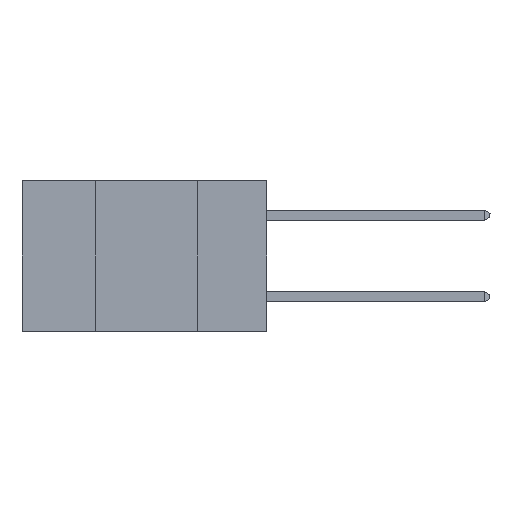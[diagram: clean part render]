
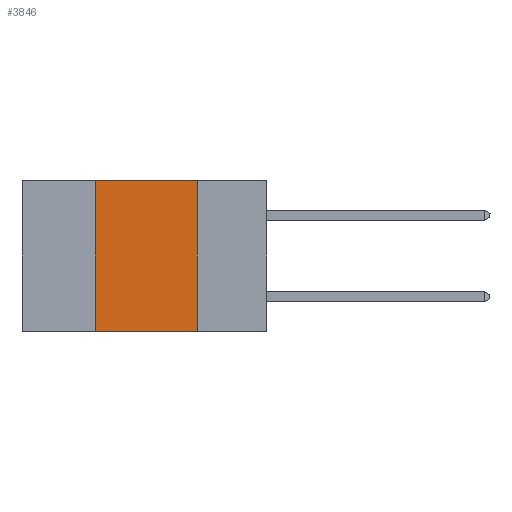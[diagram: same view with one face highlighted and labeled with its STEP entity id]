
A CAD part, left-side view. The second image highlights one B-rep face of the part: STEP entity #3846.
In plain terms, the highlighted planar face has unit normal (-1, 0, 0).
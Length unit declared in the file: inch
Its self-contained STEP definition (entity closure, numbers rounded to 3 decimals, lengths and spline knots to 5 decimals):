
#705 = VECTOR ( 'NONE', #15001, 39.37008 ) ;
#826 = PLANE ( 'NONE',  #18335 ) ;
#1712 = VECTOR ( 'NONE', #2984, 39.37008 ) ;
#1900 = DIRECTION ( 'NONE',  ( 0., -1., 0. ) ) ;
#2790 = VERTEX_POINT ( 'NONE', #8900 ) ;
#2984 = DIRECTION ( 'NONE',  ( 0., -1., 0. ) ) ;
#3592 = LINE ( 'NONE', #21150, #15235 ) ;
#3846 = ADVANCED_FACE ( 'NONE', ( #16319 ), #826, .F. ) ;
#5496 = CARTESIAN_POINT ( 'NONE',  ( 0., 0.42, 0. ) ) ;
#5572 = VERTEX_POINT ( 'NONE', #14159 ) ;
#6018 = CARTESIAN_POINT ( 'NONE',  ( 0., 0.17, 0. ) ) ;
#6295 = CARTESIAN_POINT ( 'NONE',  ( 0., 0.6, 0. ) ) ;
#7198 = LINE ( 'NONE', #5496, #8339 ) ;
#7533 = DIRECTION ( 'NONE',  ( 1., 0., 0. ) ) ;
#7712 = LINE ( 'NONE', #6018, #705 ) ;
#8339 = VECTOR ( 'NONE', #12431, 39.37008 ) ;
#8504 = CARTESIAN_POINT ( 'NONE',  ( 0., 0.42, -0.37 ) ) ;
#8900 = CARTESIAN_POINT ( 'NONE',  ( 0., 0.17, 0. ) ) ;
#9336 = EDGE_CURVE ( 'NONE', #16579, #2790, #22004, .T. ) ;
#9341 = DIRECTION ( 'NONE',  ( 0., 0., -1. ) ) ;
#10551 = CARTESIAN_POINT ( 'NONE',  ( 0., 0.42, 0. ) ) ;
#12431 = DIRECTION ( 'NONE',  ( 0., 0., 1. ) ) ;
#12897 = ORIENTED_EDGE ( 'NONE', *, *, #13171, .F. ) ;
#13171 = EDGE_CURVE ( 'NONE', #2790, #5572, #7712, .T. ) ;
#14159 = CARTESIAN_POINT ( 'NONE',  ( 0., 0.17, -0.37 ) ) ;
#14667 = EDGE_LOOP ( 'NONE', ( #12897, #15530, #20840, #14674 ) ) ;
#14674 = ORIENTED_EDGE ( 'NONE', *, *, #20108, .T. ) ;
#15001 = DIRECTION ( 'NONE',  ( 0., 0., -1. ) ) ;
#15235 = VECTOR ( 'NONE', #1900, 39.37008 ) ;
#15530 = ORIENTED_EDGE ( 'NONE', *, *, #9336, .F. ) ;
#16109 = CARTESIAN_POINT ( 'NONE',  ( 0., 0.6, 0. ) ) ;
#16319 = FACE_OUTER_BOUND ( 'NONE', #14667, .T. ) ;
#16579 = VERTEX_POINT ( 'NONE', #10551 ) ;
#17680 = VERTEX_POINT ( 'NONE', #8504 ) ;
#18335 = AXIS2_PLACEMENT_3D ( 'NONE', #16109, #7533, #9341 ) ;
#20108 = EDGE_CURVE ( 'NONE', #17680, #5572, #3592, .T. ) ;
#20840 = ORIENTED_EDGE ( 'NONE', *, *, #22460, .F. ) ;
#21150 = CARTESIAN_POINT ( 'NONE',  ( 0., 0.6, -0.37 ) ) ;
#22004 = LINE ( 'NONE', #6295, #1712 ) ;
#22460 = EDGE_CURVE ( 'NONE', #17680, #16579, #7198, .T. ) ;
